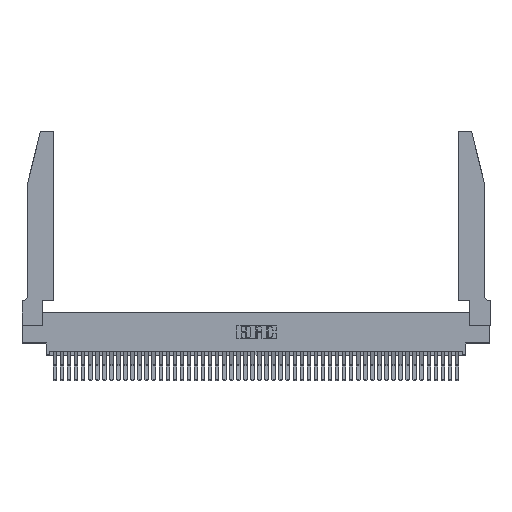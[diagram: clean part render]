
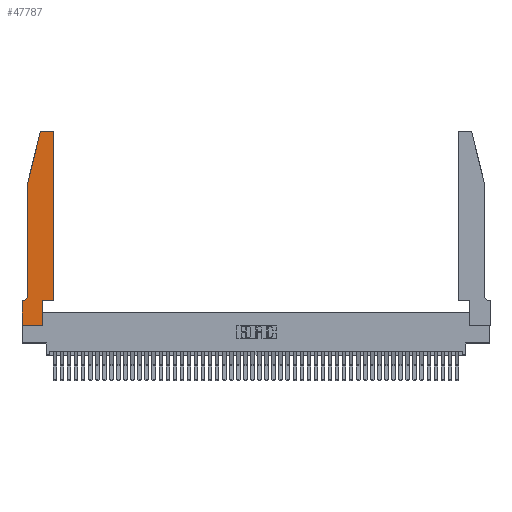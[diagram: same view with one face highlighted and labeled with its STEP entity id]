
A CAD part, top view. The second image highlights one B-rep face of the part: STEP entity #47787.
In plain terms, the highlighted planar face has unit normal (0, 0, 1).
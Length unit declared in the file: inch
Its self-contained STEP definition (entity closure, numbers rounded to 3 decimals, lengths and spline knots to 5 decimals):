
#233 = ORIENTED_EDGE ( 'NONE', *, *, #12357, .T. ) ;
#764 = CARTESIAN_POINT ( 'NONE',  ( 0.4205, 2.72, 0.37 ) ) ;
#824 = DIRECTION ( 'NONE',  ( -1., 0., 0. ) ) ;
#1444 = CARTESIAN_POINT ( 'NONE',  ( 0.4505, 0.35, 0.37 ) ) ;
#1611 = DIRECTION ( 'NONE',  ( 0., 1., 0. ) ) ;
#1676 = CARTESIAN_POINT ( 'NONE',  ( 0., 0., 0.37 ) ) ;
#2414 = ORIENTED_EDGE ( 'NONE', *, *, #17006, .T. ) ;
#3321 = LINE ( 'NONE', #28665, #41910 ) ;
#4271 = DIRECTION ( 'NONE',  ( 0., 0., 1. ) ) ;
#4511 = DIRECTION ( 'NONE',  ( 1., 0., 0. ) ) ;
#5404 = DIRECTION ( 'NONE',  ( 1., 0., 0. ) ) ;
#5437 = VECTOR ( 'NONE', #824, 39.37008 ) ;
#5499 = EDGE_CURVE ( 'NONE', #18162, #23965, #11438, .T. ) ;
#5702 = ORIENTED_EDGE ( 'NONE', *, *, #5499, .T. ) ;
#6387 = CARTESIAN_POINT ( 'NONE',  ( 0.4505, 2.72, 0.37 ) ) ;
#6731 = EDGE_CURVE ( 'NONE', #46025, #13554, #7237, .T. ) ;
#7133 = ORIENTED_EDGE ( 'NONE', *, *, #13008, .T. ) ;
#7237 = LINE ( 'NONE', #44878, #45805 ) ;
#7898 = DIRECTION ( 'NONE',  ( -0.239, -0.971, 0. ) ) ;
#8113 = LINE ( 'NONE', #29277, #35574 ) ;
#10623 = CARTESIAN_POINT ( 'NONE',  ( 0.2865, 0.35, 0.37 ) ) ;
#10629 = VERTEX_POINT ( 'NONE', #36748 ) ;
#10661 = DIRECTION ( 'NONE',  ( 0., -1., 0. ) ) ;
#10791 = EDGE_CURVE ( 'NONE', #13554, #34916, #37496, .T. ) ;
#10908 = ORIENTED_EDGE ( 'NONE', *, *, #31116, .T. ) ;
#11235 = ORIENTED_EDGE ( 'NONE', *, *, #10791, .T. ) ;
#11438 = CIRCLE ( 'NONE', #40282, 0.07 ) ;
#12357 = EDGE_CURVE ( 'NONE', #23965, #18486, #15372, .T. ) ;
#13008 = EDGE_CURVE ( 'NONE', #34916, #29319, #36938, .T. ) ;
#13202 = DIRECTION ( 'NONE',  ( 0., 0., 1. ) ) ;
#13554 = VERTEX_POINT ( 'NONE', #26347 ) ;
#14152 = EDGE_CURVE ( 'NONE', #29319, #10629, #45015, .T. ) ;
#14324 = DIRECTION ( 'NONE',  ( 0., 1., 0. ) ) ;
#15372 = LINE ( 'NONE', #26931, #5437 ) ;
#15980 = ORIENTED_EDGE ( 'NONE', *, *, #6731, .T. ) ;
#16010 = AXIS2_PLACEMENT_3D ( 'NONE', #35572, #13202, #39354 ) ;
#17006 = EDGE_CURVE ( 'NONE', #18486, #27483, #3321, .T. ) ;
#17292 = EDGE_CURVE ( 'NONE', #19230, #33995, #40113, .T. ) ;
#18087 = VECTOR ( 'NONE', #14324, 39.37008 ) ;
#18162 = VERTEX_POINT ( 'NONE', #39024 ) ;
#18486 = VERTEX_POINT ( 'NONE', #48301 ) ;
#18906 = LINE ( 'NONE', #1676, #47616 ) ;
#19230 = VERTEX_POINT ( 'NONE', #41911 ) ;
#19420 = CARTESIAN_POINT ( 'NONE',  ( 0.0055, 0.42, 0.37 ) ) ;
#19969 = ORIENTED_EDGE ( 'NONE', *, *, #17292, .T. ) ;
#20502 = PLANE ( 'NONE',  #16010 ) ;
#20681 = ORIENTED_EDGE ( 'NONE', *, *, #36492, .T. ) ;
#21941 = EDGE_CURVE ( 'NONE', #27483, #41841, #18906, .T. ) ;
#23225 = DIRECTION ( 'NONE',  ( -1., 0., 0. ) ) ;
#23363 = CARTESIAN_POINT ( 'NONE',  ( 0.0055, 0.35, 0.37 ) ) ;
#23965 = VERTEX_POINT ( 'NONE', #23363 ) ;
#25121 = VECTOR ( 'NONE', #25869, 39.37008 ) ;
#25869 = DIRECTION ( 'NONE',  ( -1., 0., 0. ) ) ;
#26347 = CARTESIAN_POINT ( 'NONE',  ( 0.4505, 0.35, 0.37 ) ) ;
#26638 = CARTESIAN_POINT ( 'NONE',  ( 0.284, 2.72, 0.37 ) ) ;
#26871 = DIRECTION ( 'NONE',  ( 0., 0., 1. ) ) ;
#26931 = CARTESIAN_POINT ( 'NONE',  ( 0.0755, 0.35, 0.37 ) ) ;
#27483 = VERTEX_POINT ( 'NONE', #47278 ) ;
#27602 = EDGE_CURVE ( 'NONE', #33995, #18162, #8113, .T. ) ;
#28063 = LINE ( 'NONE', #44108, #18087 ) ;
#28068 = EDGE_LOOP ( 'NONE', ( #43445, #20681, #19969, #30335, #5702, #233, #2414, #38693, #10908, #15980, #11235, #7133 ) ) ;
#28665 = CARTESIAN_POINT ( 'NONE',  ( 0., 0., 0.37 ) ) ;
#28877 = CARTESIAN_POINT ( 'NONE',  ( 0.4205, 2.75, 0.37 ) ) ;
#29277 = CARTESIAN_POINT ( 'NONE',  ( 0.0755, 2., 0.37 ) ) ;
#29319 = VERTEX_POINT ( 'NONE', #28877 ) ;
#30335 = ORIENTED_EDGE ( 'NONE', *, *, #27602, .T. ) ;
#30403 = DIRECTION ( 'NONE',  ( 1., 0., 0. ) ) ;
#30774 = CIRCLE ( 'NONE', #32323, 0.03 ) ;
#31116 = EDGE_CURVE ( 'NONE', #41841, #46025, #28063, .T. ) ;
#32323 = AXIS2_PLACEMENT_3D ( 'NONE', #26638, #4271, #30403 ) ;
#33238 = AXIS2_PLACEMENT_3D ( 'NONE', #764, #26871, #4511 ) ;
#33736 = DIRECTION ( 'NONE',  ( 1., 0., 0. ) ) ;
#33891 = CARTESIAN_POINT ( 'NONE',  ( 0.2865, 0., 0.37 ) ) ;
#33995 = VERTEX_POINT ( 'NONE', #38570 ) ;
#34916 = VERTEX_POINT ( 'NONE', #6387 ) ;
#35572 = CARTESIAN_POINT ( 'NONE',  ( 0., 0.35, 0.37 ) ) ;
#35574 = VECTOR ( 'NONE', #10661, 39.37008 ) ;
#36492 = EDGE_CURVE ( 'NONE', #10629, #19230, #30774, .T. ) ;
#36748 = CARTESIAN_POINT ( 'NONE',  ( 0.284, 2.75, 0.37 ) ) ;
#36938 = CIRCLE ( 'NONE', #33238, 0.03 ) ;
#37374 = FACE_OUTER_BOUND ( 'NONE', #28068, .T. ) ;
#37496 = LINE ( 'NONE', #1444, #47233 ) ;
#37628 = CARTESIAN_POINT ( 'NONE',  ( 0.0755, 2., 0.37 ) ) ;
#38570 = CARTESIAN_POINT ( 'NONE',  ( 0.0755, 2., 0.37 ) ) ;
#38693 = ORIENTED_EDGE ( 'NONE', *, *, #21941, .T. ) ;
#38922 = VECTOR ( 'NONE', #7898, 39.37008 ) ;
#39024 = CARTESIAN_POINT ( 'NONE',  ( 0.0755, 0.42, 0.37 ) ) ;
#39354 = DIRECTION ( 'NONE',  ( 1., 0., 0. ) ) ;
#39953 = DIRECTION ( 'NONE',  ( 0., -1., 0. ) ) ;
#40113 = LINE ( 'NONE', #37628, #38922 ) ;
#40282 = AXIS2_PLACEMENT_3D ( 'NONE', #19420, #45626, #23225 ) ;
#41841 = VERTEX_POINT ( 'NONE', #33891 ) ;
#41910 = VECTOR ( 'NONE', #39953, 39.37008 ) ;
#41911 = CARTESIAN_POINT ( 'NONE',  ( 0.25487, 2.72718, 0.37 ) ) ;
#43445 = ORIENTED_EDGE ( 'NONE', *, *, #14152, .T. ) ;
#44108 = CARTESIAN_POINT ( 'NONE',  ( 0.2865, 0.35, 0.37 ) ) ;
#44360 = CARTESIAN_POINT ( 'NONE',  ( 0.2605, 2.75, 0.37 ) ) ;
#44878 = CARTESIAN_POINT ( 'NONE',  ( 0.4505, 0.35, 0.37 ) ) ;
#45015 = LINE ( 'NONE', #44360, #25121 ) ;
#45626 = DIRECTION ( 'NONE',  ( 0., 0., -1. ) ) ;
#45805 = VECTOR ( 'NONE', #33736, 39.37008 ) ;
#46025 = VERTEX_POINT ( 'NONE', #10623 ) ;
#47233 = VECTOR ( 'NONE', #1611, 39.37008 ) ;
#47278 = CARTESIAN_POINT ( 'NONE',  ( 0., 0., 0.37 ) ) ;
#47616 = VECTOR ( 'NONE', #5404, 39.37008 ) ;
#47787 = ADVANCED_FACE ( 'NONE', ( #37374 ), #20502, .T. ) ;
#48301 = CARTESIAN_POINT ( 'NONE',  ( 0., 0.35, 0.37 ) ) ;
